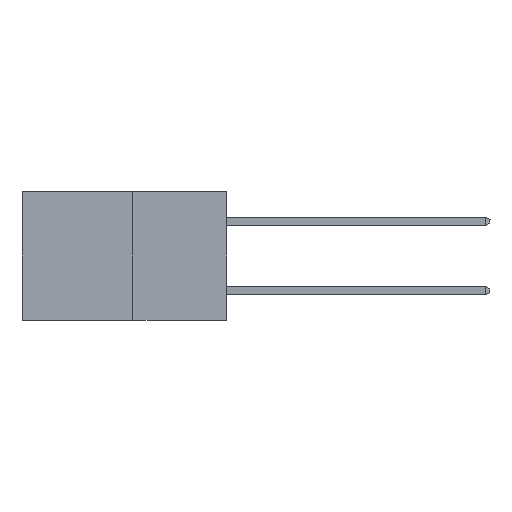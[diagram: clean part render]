
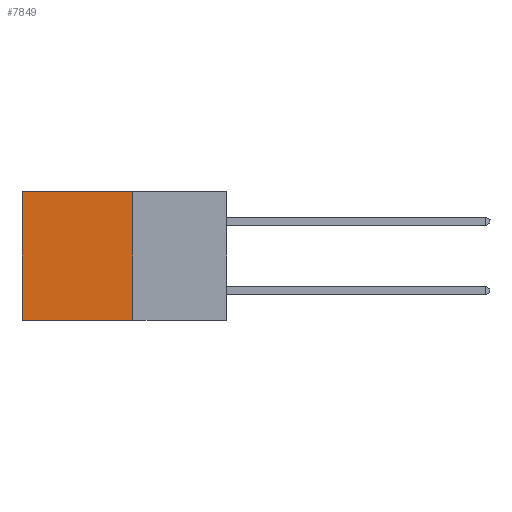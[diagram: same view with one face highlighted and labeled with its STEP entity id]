
A CAD part, left-side view. The second image highlights one B-rep face of the part: STEP entity #7849.
In plain terms, the highlighted planar face has unit normal (-1, 0, 0).
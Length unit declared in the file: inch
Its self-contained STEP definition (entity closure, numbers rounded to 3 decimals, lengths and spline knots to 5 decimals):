
#226 = DIRECTION ( 'NONE',  ( 0., 1., 0. ) ) ;
#604 = VECTOR ( 'NONE', #226, 39.37008 ) ;
#733 = CARTESIAN_POINT ( 'NONE',  ( 0.277, 0.59, 0. ) ) ;
#1225 = EDGE_CURVE ( 'NONE', #13788, #14715, #8837, .T. ) ;
#1518 = VECTOR ( 'NONE', #7265, 39.37008 ) ;
#1874 = ORIENTED_EDGE ( 'NONE', *, *, #1225, .T. ) ;
#2180 = CARTESIAN_POINT ( 'NONE',  ( 0.277, 0.27, -0.37 ) ) ;
#2306 = CARTESIAN_POINT ( 'NONE',  ( 0.277, 0.59, -0.37 ) ) ;
#2320 = VECTOR ( 'NONE', #12712, 39.37008 ) ;
#2483 = AXIS2_PLACEMENT_3D ( 'NONE', #2180, #5593, #13644 ) ;
#2576 = ORIENTED_EDGE ( 'NONE', *, *, #3036, .F. ) ;
#3036 = EDGE_CURVE ( 'NONE', #6541, #13129, #11471, .T. ) ;
#4847 = ORIENTED_EDGE ( 'NONE', *, *, #13042, .F. ) ;
#5588 = ORIENTED_EDGE ( 'NONE', *, *, #7333, .T. ) ;
#5593 = DIRECTION ( 'NONE',  ( 1., 0., 0. ) ) ;
#5814 = CARTESIAN_POINT ( 'NONE',  ( 0.277, 0.27, 0. ) ) ;
#6541 = VERTEX_POINT ( 'NONE', #6784 ) ;
#6784 = CARTESIAN_POINT ( 'NONE',  ( 0.277, 0.27, 0. ) ) ;
#7265 = DIRECTION ( 'NONE',  ( 0., 1., 0. ) ) ;
#7333 = EDGE_CURVE ( 'NONE', #6541, #13788, #12763, .T. ) ;
#7735 = EDGE_LOOP ( 'NONE', ( #1874, #4847, #2576, #5588 ) ) ;
#7849 = ADVANCED_FACE ( 'NONE', ( #12381 ), #12496, .F. ) ;
#8837 = LINE ( 'NONE', #13822, #14528 ) ;
#10278 = LINE ( 'NONE', #14160, #1518 ) ;
#11471 = LINE ( 'NONE', #12681, #2320 ) ;
#12381 = FACE_OUTER_BOUND ( 'NONE', #7735, .T. ) ;
#12496 = PLANE ( 'NONE',  #2483 ) ;
#12681 = CARTESIAN_POINT ( 'NONE',  ( 0.277, 0.27, -0.37 ) ) ;
#12712 = DIRECTION ( 'NONE',  ( 0., 0., -1. ) ) ;
#12763 = LINE ( 'NONE', #5814, #604 ) ;
#12966 = DIRECTION ( 'NONE',  ( 0., 0., -1. ) ) ;
#13042 = EDGE_CURVE ( 'NONE', #13129, #14715, #10278, .T. ) ;
#13129 = VERTEX_POINT ( 'NONE', #13161 ) ;
#13161 = CARTESIAN_POINT ( 'NONE',  ( 0.277, 0.27, -0.37 ) ) ;
#13644 = DIRECTION ( 'NONE',  ( 0., 0., -1. ) ) ;
#13788 = VERTEX_POINT ( 'NONE', #733 ) ;
#13822 = CARTESIAN_POINT ( 'NONE',  ( 0.277, 0.59, -0.37 ) ) ;
#14160 = CARTESIAN_POINT ( 'NONE',  ( 0.277, 0.27, -0.37 ) ) ;
#14528 = VECTOR ( 'NONE', #12966, 39.37008 ) ;
#14715 = VERTEX_POINT ( 'NONE', #2306 ) ;
